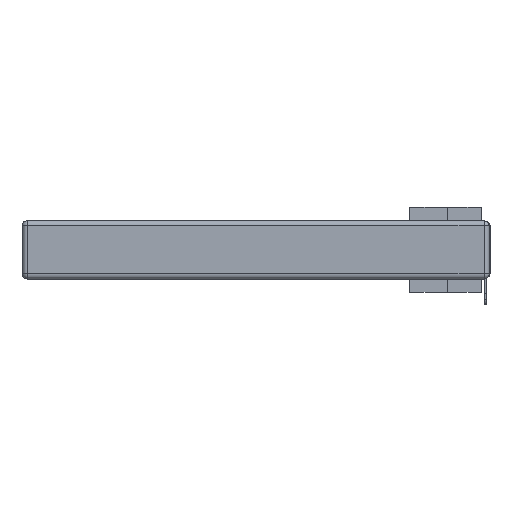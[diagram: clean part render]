
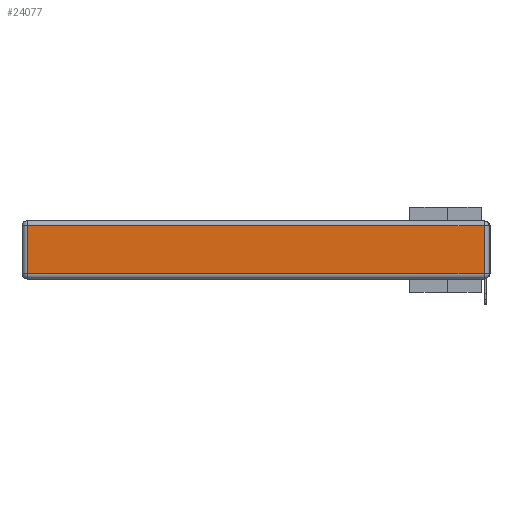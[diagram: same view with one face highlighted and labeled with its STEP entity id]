
A CAD part, left-side view. The second image highlights one B-rep face of the part: STEP entity #24077.
In plain terms, the highlighted planar face has unit normal (-1, 0, 0).
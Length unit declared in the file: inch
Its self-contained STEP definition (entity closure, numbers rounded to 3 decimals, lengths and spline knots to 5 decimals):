
#400 = EDGE_CURVE ( 'NONE', #22244, #14370, #24814, .T. ) ;
#517 = CARTESIAN_POINT ( 'NONE',  ( 0., 0., -0.313 ) ) ;
#527 = EDGE_LOOP ( 'NONE', ( #24948, #34115, #13612, #8395 ) ) ;
#1565 = FACE_OUTER_BOUND ( 'NONE', #527, .T. ) ;
#2306 = LINE ( 'NONE', #29502, #3002 ) ;
#3002 = VECTOR ( 'NONE', #35807, 39.37008 ) ;
#3922 = DIRECTION ( 'NONE',  ( 0., 1., 0. ) ) ;
#4543 = DIRECTION ( 'NONE',  ( 0., 0., -1. ) ) ;
#4723 = CARTESIAN_POINT ( 'NONE',  ( 0., 0., -0.343 ) ) ;
#5504 = VECTOR ( 'NONE', #4543, 39.37008 ) ;
#6527 = LINE ( 'NONE', #11654, #5504 ) ;
#8395 = ORIENTED_EDGE ( 'NONE', *, *, #16840, .T. ) ;
#9405 = LINE ( 'NONE', #517, #28072 ) ;
#10218 = VERTEX_POINT ( 'NONE', #11922 ) ;
#10519 = VERTEX_POINT ( 'NONE', #29033 ) ;
#11654 = CARTESIAN_POINT ( 'NONE',  ( 0., 2.72, -0.343 ) ) ;
#11746 = VECTOR ( 'NONE', #3922, 39.37008 ) ;
#11922 = CARTESIAN_POINT ( 'NONE',  ( 0., 0.03, -0.313 ) ) ;
#13612 = ORIENTED_EDGE ( 'NONE', *, *, #400, .T. ) ;
#13776 = DIRECTION ( 'NONE',  ( 0., 0., 1. ) ) ;
#14370 = VERTEX_POINT ( 'NONE', #28915 ) ;
#15717 = EDGE_CURVE ( 'NONE', #10218, #22244, #2306, .T. ) ;
#15823 = AXIS2_PLACEMENT_3D ( 'NONE', #4723, #25614, #13776 ) ;
#16840 = EDGE_CURVE ( 'NONE', #14370, #10519, #6527, .T. ) ;
#19106 = PLANE ( 'NONE',  #15823 ) ;
#21500 = CARTESIAN_POINT ( 'NONE',  ( 0., 0.03, -0.03 ) ) ;
#22244 = VERTEX_POINT ( 'NONE', #21500 ) ;
#24077 = ADVANCED_FACE ( 'NONE', ( #1565 ), #19106, .T. ) ;
#24424 = CARTESIAN_POINT ( 'NONE',  ( 0., 2.75, -0.03 ) ) ;
#24814 = LINE ( 'NONE', #24424, #11746 ) ;
#24948 = ORIENTED_EDGE ( 'NONE', *, *, #31536, .T. ) ;
#25614 = DIRECTION ( 'NONE',  ( -1., 0., 0. ) ) ;
#28072 = VECTOR ( 'NONE', #33266, 39.37008 ) ;
#28915 = CARTESIAN_POINT ( 'NONE',  ( 0., 2.72, -0.03 ) ) ;
#29033 = CARTESIAN_POINT ( 'NONE',  ( 0., 2.72, -0.313 ) ) ;
#29502 = CARTESIAN_POINT ( 'NONE',  ( 0., 0.03, -0.343 ) ) ;
#31536 = EDGE_CURVE ( 'NONE', #10519, #10218, #9405, .T. ) ;
#33266 = DIRECTION ( 'NONE',  ( 0., -1., 0. ) ) ;
#34115 = ORIENTED_EDGE ( 'NONE', *, *, #15717, .T. ) ;
#35807 = DIRECTION ( 'NONE',  ( 0., 0., 1. ) ) ;
